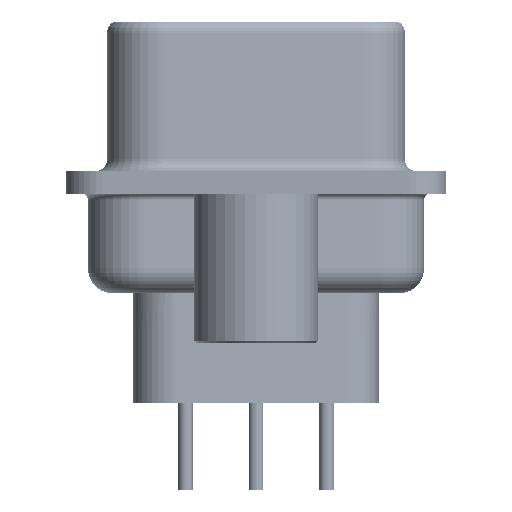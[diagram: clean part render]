
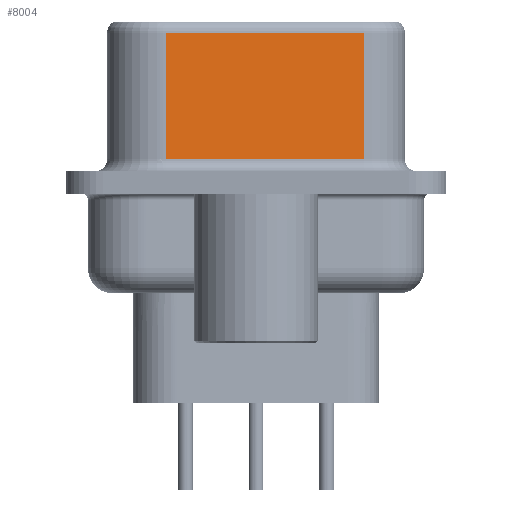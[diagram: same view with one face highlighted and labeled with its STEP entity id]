
A CAD part, left-side view. The second image highlights one B-rep face of the part: STEP entity #8004.
In plain terms, the highlighted planar face has unit normal (-0.985, -0.174, 0).
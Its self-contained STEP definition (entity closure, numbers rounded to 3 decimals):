
#2617 = VERTEX_POINT ( 'NONE', #8080 ) ;
#2978 = FACE_OUTER_BOUND ( 'NONE', #11264, .T. ) ;
#3091 = LINE ( 'NONE', #15029, #22593 ) ;
#5854 = CARTESIAN_POINT ( 'NONE',  ( 5.132, -4.322, 6.52 ) ) ;
#6279 = DIRECTION ( 'NONE',  ( -0.174, 0.985, 0. ) ) ;
#8004 = ADVANCED_FACE ( 'NONE', ( #2978 ), #34421, .F. ) ;
#8080 = CARTESIAN_POINT ( 'NONE',  ( 5.132, -4.322, 0.95 ) ) ;
#8155 = CARTESIAN_POINT ( 'NONE',  ( 5.132, -4.322, 6.02 ) ) ;
#11264 = EDGE_LOOP ( 'NONE', ( #31817, #19221, #32130, #21469 ) ) ;
#12267 = EDGE_CURVE ( 'NONE', #23226, #27051, #21944, .T. ) ;
#12525 = VECTOR ( 'NONE', #21540, 1000. ) ;
#13360 = VECTOR ( 'NONE', #36912, 1000. ) ;
#13399 = DIRECTION ( 'NONE',  ( 0., 0., -1. ) ) ;
#15029 = CARTESIAN_POINT ( 'NONE',  ( 5.132, -4.322, 0.95 ) ) ;
#15140 = CARTESIAN_POINT ( 'NONE',  ( 3.73, 3.628, 6.52 ) ) ;
#15653 = DIRECTION ( 'NONE',  ( 0.174, -0.985, 0. ) ) ;
#17621 = LINE ( 'NONE', #8155, #13360 ) ;
#18814 = EDGE_CURVE ( 'NONE', #20419, #23226, #17621, .T. ) ;
#19221 = ORIENTED_EDGE ( 'NONE', *, *, #18814, .T. ) ;
#19280 = EDGE_CURVE ( 'NONE', #27051, #2617, #3091, .T. ) ;
#20419 = VERTEX_POINT ( 'NONE', #27087 ) ;
#21469 = ORIENTED_EDGE ( 'NONE', *, *, #19280, .T. ) ;
#21540 = DIRECTION ( 'NONE',  ( 0., 0., -1. ) ) ;
#21790 = CARTESIAN_POINT ( 'NONE',  ( 3.73, 3.628, 6.02 ) ) ;
#21944 = LINE ( 'NONE', #15140, #12525 ) ;
#22267 = CARTESIAN_POINT ( 'NONE',  ( 5.132, -4.322, 6.52 ) ) ;
#22593 = VECTOR ( 'NONE', #15653, 1000. ) ;
#23226 = VERTEX_POINT ( 'NONE', #21790 ) ;
#27051 = VERTEX_POINT ( 'NONE', #32396 ) ;
#27087 = CARTESIAN_POINT ( 'NONE',  ( 5.132, -4.322, 6.02 ) ) ;
#29584 = VECTOR ( 'NONE', #13399, 1000. ) ;
#31817 = ORIENTED_EDGE ( 'NONE', *, *, #37852, .F. ) ;
#32095 = LINE ( 'NONE', #22267, #29584 ) ;
#32130 = ORIENTED_EDGE ( 'NONE', *, *, #12267, .T. ) ;
#32396 = CARTESIAN_POINT ( 'NONE',  ( 3.73, 3.628, 0.95 ) ) ;
#34421 = PLANE ( 'NONE',  #39133 ) ;
#36912 = DIRECTION ( 'NONE',  ( -0.174, 0.985, 0. ) ) ;
#37852 = EDGE_CURVE ( 'NONE', #20419, #2617, #32095, .T. ) ;
#37925 = DIRECTION ( 'NONE',  ( 0.985, 0.174, 0. ) ) ;
#39133 = AXIS2_PLACEMENT_3D ( 'NONE', #5854, #37925, #6279 ) ;
